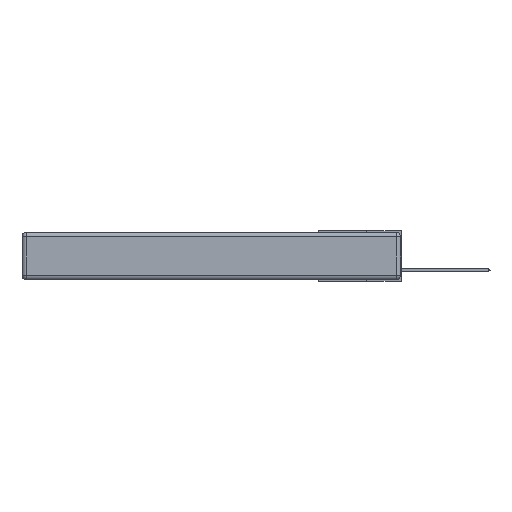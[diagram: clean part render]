
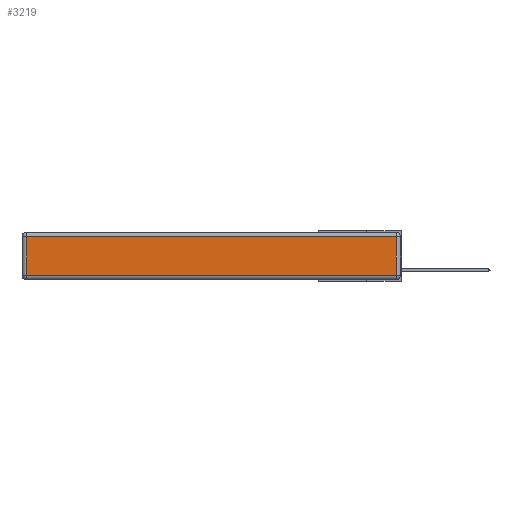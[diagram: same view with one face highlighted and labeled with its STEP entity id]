
A CAD part, left-side view. The second image highlights one B-rep face of the part: STEP entity #3219.
In plain terms, the highlighted planar face has unit normal (-1, 0, 0).
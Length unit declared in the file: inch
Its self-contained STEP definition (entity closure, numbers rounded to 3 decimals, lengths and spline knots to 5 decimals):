
#81 = VECTOR ( 'NONE', #14519, 39.37008 ) ;
#1552 = LINE ( 'NONE', #27102, #14673 ) ;
#1650 = VERTEX_POINT ( 'NONE', #9882 ) ;
#2401 = VECTOR ( 'NONE', #4381, 39.37008 ) ;
#3023 = DIRECTION ( 'NONE',  ( 0., 1., 0. ) ) ;
#3219 = ADVANCED_FACE ( 'NONE', ( #9642 ), #8549, .T. ) ;
#3347 = DIRECTION ( 'NONE',  ( -1., 0., 0. ) ) ;
#3767 = VECTOR ( 'NONE', #21964, 39.37008 ) ;
#4336 = EDGE_CURVE ( 'NONE', #28199, #19199, #7090, .T. ) ;
#4381 = DIRECTION ( 'NONE',  ( 0., 0., 1. ) ) ;
#5997 = DIRECTION ( 'NONE',  ( 0., 0., 1. ) ) ;
#7090 = LINE ( 'NONE', #22349, #81 ) ;
#7772 = CARTESIAN_POINT ( 'NONE',  ( 0., 2.72, -0.03 ) ) ;
#7893 = CARTESIAN_POINT ( 'NONE',  ( 0., 0.03, -0.313 ) ) ;
#8549 = PLANE ( 'NONE',  #29378 ) ;
#8558 = ORIENTED_EDGE ( 'NONE', *, *, #20401, .T. ) ;
#9642 = FACE_OUTER_BOUND ( 'NONE', #26227, .T. ) ;
#9882 = CARTESIAN_POINT ( 'NONE',  ( 0., 0.03, -0.03 ) ) ;
#10659 = VERTEX_POINT ( 'NONE', #7893 ) ;
#12899 = EDGE_CURVE ( 'NONE', #19199, #10659, #33714, .T. ) ;
#13776 = CARTESIAN_POINT ( 'NONE',  ( 0., 0., -0.343 ) ) ;
#14519 = DIRECTION ( 'NONE',  ( 0., 0., -1. ) ) ;
#14673 = VECTOR ( 'NONE', #3023, 39.37008 ) ;
#15637 = CARTESIAN_POINT ( 'NONE',  ( 0., 2.72, -0.313 ) ) ;
#17063 = ORIENTED_EDGE ( 'NONE', *, *, #12899, .T. ) ;
#17426 = CARTESIAN_POINT ( 'NONE',  ( 0., 0.03, -0.343 ) ) ;
#19199 = VERTEX_POINT ( 'NONE', #15637 ) ;
#19673 = ORIENTED_EDGE ( 'NONE', *, *, #19977, .T. ) ;
#19977 = EDGE_CURVE ( 'NONE', #10659, #1650, #31968, .T. ) ;
#20401 = EDGE_CURVE ( 'NONE', #1650, #28199, #1552, .T. ) ;
#21964 = DIRECTION ( 'NONE',  ( 0., -1., 0. ) ) ;
#22349 = CARTESIAN_POINT ( 'NONE',  ( 0., 2.72, -0.343 ) ) ;
#26227 = EDGE_LOOP ( 'NONE', ( #17063, #19673, #8558, #33201 ) ) ;
#26768 = CARTESIAN_POINT ( 'NONE',  ( 0., 0., -0.313 ) ) ;
#27102 = CARTESIAN_POINT ( 'NONE',  ( 0., 2.75, -0.03 ) ) ;
#28199 = VERTEX_POINT ( 'NONE', #7772 ) ;
#29378 = AXIS2_PLACEMENT_3D ( 'NONE', #13776, #3347, #5997 ) ;
#31968 = LINE ( 'NONE', #17426, #2401 ) ;
#33201 = ORIENTED_EDGE ( 'NONE', *, *, #4336, .T. ) ;
#33714 = LINE ( 'NONE', #26768, #3767 ) ;
